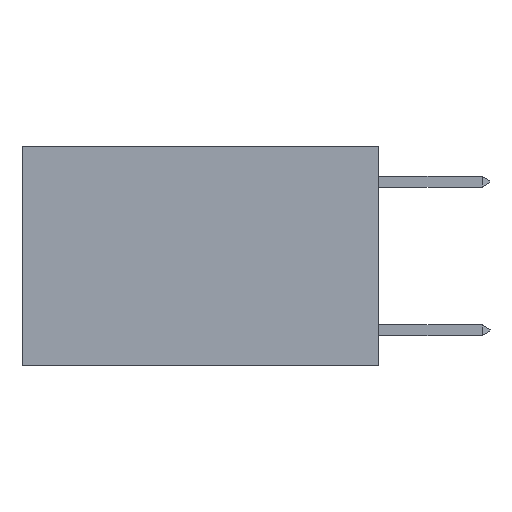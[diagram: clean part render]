
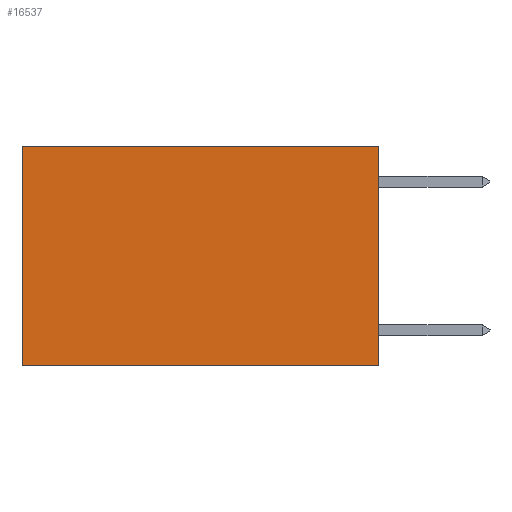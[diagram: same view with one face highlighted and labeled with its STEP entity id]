
A CAD part, left-side view. The second image highlights one B-rep face of the part: STEP entity #16537.
In plain terms, the highlighted planar face has unit normal (-1, 0, 0).
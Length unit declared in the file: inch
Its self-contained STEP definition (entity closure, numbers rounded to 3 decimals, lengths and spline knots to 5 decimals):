
#77 = ORIENTED_EDGE ( 'NONE', *, *, #9597, .F. ) ;
#143 = CARTESIAN_POINT ( 'NONE',  ( 0.2625, 0., -0.37 ) ) ;
#305 = EDGE_CURVE ( 'NONE', #17482, #14537, #4769, .T. ) ;
#409 = VECTOR ( 'NONE', #11261, 39.37008 ) ;
#453 = DIRECTION ( 'NONE',  ( 0., 1., 0. ) ) ;
#926 = CARTESIAN_POINT ( 'NONE',  ( 0.2625, 0.6, 0. ) ) ;
#1023 = EDGE_CURVE ( 'NONE', #2204, #14537, #14580, .T. ) ;
#1418 = VECTOR ( 'NONE', #18135, 39.37008 ) ;
#2204 = VERTEX_POINT ( 'NONE', #926 ) ;
#3065 = CARTESIAN_POINT ( 'NONE',  ( 0.2625, 0.6, -0.37 ) ) ;
#3347 = EDGE_LOOP ( 'NONE', ( #7189, #15598, #77, #13128 ) ) ;
#4769 = LINE ( 'NONE', #143, #1418 ) ;
#7189 = ORIENTED_EDGE ( 'NONE', *, *, #1023, .T. ) ;
#7423 = VECTOR ( 'NONE', #9088, 39.37008 ) ;
#8037 = LINE ( 'NONE', #8352, #409 ) ;
#8352 = CARTESIAN_POINT ( 'NONE',  ( 0.2625, 0., 0. ) ) ;
#8361 = CARTESIAN_POINT ( 'NONE',  ( 0.2625, 0., -0.37 ) ) ;
#8688 = DIRECTION ( 'NONE',  ( 0., 0., -1. ) ) ;
#9052 = VERTEX_POINT ( 'NONE', #11394 ) ;
#9088 = DIRECTION ( 'NONE',  ( 0., 0., -1. ) ) ;
#9597 = EDGE_CURVE ( 'NONE', #9052, #17482, #8037, .T. ) ;
#9669 = VECTOR ( 'NONE', #453, 39.37008 ) ;
#10091 = CARTESIAN_POINT ( 'NONE',  ( 0.2625, 0., 0. ) ) ;
#10107 = LINE ( 'NONE', #13282, #9669 ) ;
#11261 = DIRECTION ( 'NONE',  ( 0., 0., -1. ) ) ;
#11394 = CARTESIAN_POINT ( 'NONE',  ( 0.2625, 0., 0. ) ) ;
#13128 = ORIENTED_EDGE ( 'NONE', *, *, #14051, .T. ) ;
#13282 = CARTESIAN_POINT ( 'NONE',  ( 0.2625, 0., 0. ) ) ;
#14051 = EDGE_CURVE ( 'NONE', #9052, #2204, #10107, .T. ) ;
#14181 = CARTESIAN_POINT ( 'NONE',  ( 0.2625, 0.6, 0. ) ) ;
#14537 = VERTEX_POINT ( 'NONE', #3065 ) ;
#14580 = LINE ( 'NONE', #14181, #7423 ) ;
#14730 = AXIS2_PLACEMENT_3D ( 'NONE', #10091, #17232, #8688 ) ;
#15598 = ORIENTED_EDGE ( 'NONE', *, *, #305, .F. ) ;
#15814 = PLANE ( 'NONE',  #14730 ) ;
#16537 = ADVANCED_FACE ( 'NONE', ( #16555 ), #15814, .F. ) ;
#16555 = FACE_OUTER_BOUND ( 'NONE', #3347, .T. ) ;
#17232 = DIRECTION ( 'NONE',  ( 1., 0., 0. ) ) ;
#17482 = VERTEX_POINT ( 'NONE', #8361 ) ;
#18135 = DIRECTION ( 'NONE',  ( 0., 1., 0. ) ) ;
